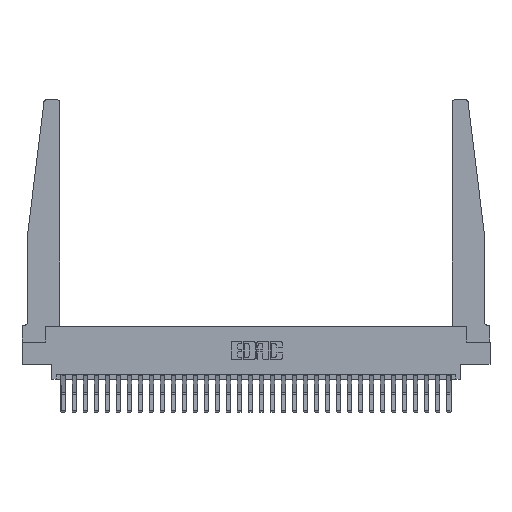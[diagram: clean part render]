
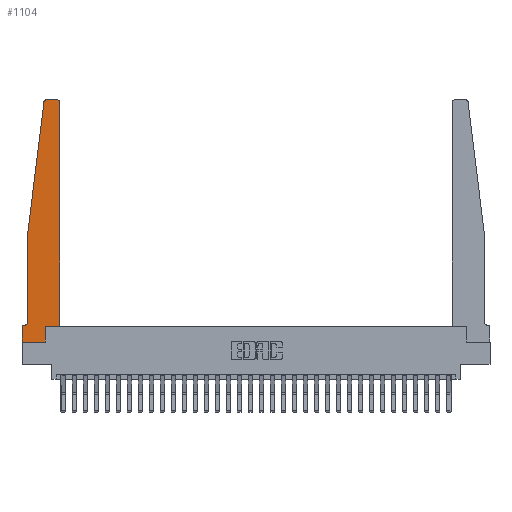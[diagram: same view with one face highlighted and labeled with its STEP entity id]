
A CAD part, top view. The second image highlights one B-rep face of the part: STEP entity #1104.
In plain terms, the highlighted planar face has unit normal (0, 0, 1).
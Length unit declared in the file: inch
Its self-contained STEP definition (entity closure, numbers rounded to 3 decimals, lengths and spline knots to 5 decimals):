
#281 = VERTEX_POINT ( 'NONE', #12625 ) ;
#428 = CARTESIAN_POINT ( 'NONE',  ( 0.425, 0.18, 0.37 ) ) ;
#993 = VECTOR ( 'NONE', #18724, 39.37008 ) ;
#1104 = ADVANCED_FACE ( 'NONE', ( #3793 ), #6349, .T. ) ;
#2392 = CARTESIAN_POINT ( 'NONE',  ( 0.425, 0.18, 0.37 ) ) ;
#2887 = VERTEX_POINT ( 'NONE', #12750 ) ;
#3393 = EDGE_CURVE ( 'NONE', #4635, #18108, #15848, .T. ) ;
#3676 = AXIS2_PLACEMENT_3D ( 'NONE', #27853, #23780, #19099 ) ;
#3747 = VERTEX_POINT ( 'NONE', #24875 ) ;
#3793 = FACE_OUTER_BOUND ( 'NONE', #11857, .T. ) ;
#3943 = DIRECTION ( 'NONE',  ( 0., 0., 1. ) ) ;
#4390 = AXIS2_PLACEMENT_3D ( 'NONE', #8921, #13291, #22461 ) ;
#4431 = CARTESIAN_POINT ( 'NONE',  ( 0.395, 2.75, 0.37 ) ) ;
#4555 = ORIENTED_EDGE ( 'NONE', *, *, #25741, .T. ) ;
#4635 = VERTEX_POINT ( 'NONE', #4431 ) ;
#4851 = ORIENTED_EDGE ( 'NONE', *, *, #26633, .T. ) ;
#4952 = LINE ( 'NONE', #2392, #10342 ) ;
#5190 = CARTESIAN_POINT ( 'NONE',  ( 0.24675, 2.72367, 0.37 ) ) ;
#5526 = EDGE_CURVE ( 'NONE', #20785, #5981, #12015, .T. ) ;
#5564 = EDGE_CURVE ( 'NONE', #19198, #20785, #4952, .T. ) ;
#5981 = VERTEX_POINT ( 'NONE', #10165 ) ;
#6349 = PLANE ( 'NONE',  #9485 ) ;
#6822 = ORIENTED_EDGE ( 'NONE', *, *, #18999, .T. ) ;
#6981 = EDGE_CURVE ( 'NONE', #5981, #4635, #8471, .T. ) ;
#7064 = ORIENTED_EDGE ( 'NONE', *, *, #13809, .T. ) ;
#7078 = CARTESIAN_POINT ( 'NONE',  ( 0., 0., 0.37 ) ) ;
#7218 = LINE ( 'NONE', #16685, #26834 ) ;
#7412 = DIRECTION ( 'NONE',  ( 0., 1., 0. ) ) ;
#7441 = VECTOR ( 'NONE', #9609, 39.37008 ) ;
#7680 = ORIENTED_EDGE ( 'NONE', *, *, #20753, .T. ) ;
#8471 = CIRCLE ( 'NONE', #21448, 0.03 ) ;
#8921 = CARTESIAN_POINT ( 'NONE',  ( 0.27653, 2.72, 0.37 ) ) ;
#9253 = CARTESIAN_POINT ( 'NONE',  ( 0.065, 0.1875, 0.37 ) ) ;
#9485 = AXIS2_PLACEMENT_3D ( 'NONE', #10552, #13115, #26671 ) ;
#9609 = DIRECTION ( 'NONE',  ( 0., 1., 0. ) ) ;
#10165 = CARTESIAN_POINT ( 'NONE',  ( 0.425, 2.72, 0.37 ) ) ;
#10342 = VECTOR ( 'NONE', #27972, 39.37008 ) ;
#10552 = CARTESIAN_POINT ( 'NONE',  ( 0., 0.1875, 0.37 ) ) ;
#10555 = VECTOR ( 'NONE', #16249, 39.37008 ) ;
#10587 = VECTOR ( 'NONE', #17979, 39.37008 ) ;
#11857 = EDGE_LOOP ( 'NONE', ( #19240, #20415, #21655, #7064, #7680, #23654, #4851, #4555, #6822, #20769, #21695, #27498 ) ) ;
#12015 = LINE ( 'NONE', #428, #7441 ) ;
#12625 = CARTESIAN_POINT ( 'NONE',  ( 0.065, 0.2375, 0.37 ) ) ;
#12696 = VERTEX_POINT ( 'NONE', #20970 ) ;
#12750 = CARTESIAN_POINT ( 'NONE',  ( 0.2605, 0., 0.37 ) ) ;
#13115 = DIRECTION ( 'NONE',  ( 0., 0., 1. ) ) ;
#13291 = DIRECTION ( 'NONE',  ( 0., 0., 1. ) ) ;
#13411 = CARTESIAN_POINT ( 'NONE',  ( 0.395, 2.72, 0.37 ) ) ;
#13669 = CARTESIAN_POINT ( 'NONE',  ( 0.27653, 2.75, 0.37 ) ) ;
#13781 = VECTOR ( 'NONE', #15879, 39.37008 ) ;
#13809 = EDGE_CURVE ( 'NONE', #14260, #281, #16159, .T. ) ;
#14064 = LINE ( 'NONE', #27769, #993 ) ;
#14260 = VERTEX_POINT ( 'NONE', #25905 ) ;
#14489 = VERTEX_POINT ( 'NONE', #16757 ) ;
#14740 = EDGE_CURVE ( 'NONE', #18108, #15865, #15899, .T. ) ;
#15848 = LINE ( 'NONE', #27013, #23288 ) ;
#15865 = VERTEX_POINT ( 'NONE', #5190 ) ;
#15879 = DIRECTION ( 'NONE',  ( -1., 0., 0. ) ) ;
#15899 = CIRCLE ( 'NONE', #4390, 0.03 ) ;
#16159 = LINE ( 'NONE', #22499, #10587 ) ;
#16249 = DIRECTION ( 'NONE',  ( 0., -1., 0. ) ) ;
#16637 = CIRCLE ( 'NONE', #3676, 0.05 ) ;
#16685 = CARTESIAN_POINT ( 'NONE',  ( 0.065, 1.25, 0.37 ) ) ;
#16757 = CARTESIAN_POINT ( 'NONE',  ( 0., 0.1875, 0.37 ) ) ;
#16879 = CARTESIAN_POINT ( 'NONE',  ( 0.2605, 0.18, 0.37 ) ) ;
#17979 = DIRECTION ( 'NONE',  ( 0., -1., 0. ) ) ;
#18108 = VERTEX_POINT ( 'NONE', #13669 ) ;
#18135 = LINE ( 'NONE', #9253, #13781 ) ;
#18724 = DIRECTION ( 'NONE',  ( 1., 0., 0. ) ) ;
#18999 = EDGE_CURVE ( 'NONE', #2887, #19198, #25777, .T. ) ;
#19099 = DIRECTION ( 'NONE',  ( -1., 0., 0. ) ) ;
#19198 = VERTEX_POINT ( 'NONE', #28633 ) ;
#19240 = ORIENTED_EDGE ( 'NONE', *, *, #3393, .T. ) ;
#20415 = ORIENTED_EDGE ( 'NONE', *, *, #14740, .T. ) ;
#20753 = EDGE_CURVE ( 'NONE', #281, #3747, #16637, .T. ) ;
#20769 = ORIENTED_EDGE ( 'NONE', *, *, #5564, .T. ) ;
#20785 = VERTEX_POINT ( 'NONE', #21368 ) ;
#20970 = CARTESIAN_POINT ( 'NONE',  ( 0., 0., 0.37 ) ) ;
#21368 = CARTESIAN_POINT ( 'NONE',  ( 0.425, 0.18, 0.37 ) ) ;
#21448 = AXIS2_PLACEMENT_3D ( 'NONE', #13411, #3943, #22140 ) ;
#21483 = EDGE_CURVE ( 'NONE', #3747, #14489, #18135, .T. ) ;
#21655 = ORIENTED_EDGE ( 'NONE', *, *, #23556, .T. ) ;
#21695 = ORIENTED_EDGE ( 'NONE', *, *, #5526, .T. ) ;
#22140 = DIRECTION ( 'NONE',  ( 1., 0., 0. ) ) ;
#22461 = DIRECTION ( 'NONE',  ( 1., 0., 0. ) ) ;
#22499 = CARTESIAN_POINT ( 'NONE',  ( 0.065, 1.25, 0.37 ) ) ;
#23288 = VECTOR ( 'NONE', #29114, 39.37008 ) ;
#23556 = EDGE_CURVE ( 'NONE', #15865, #14260, #7218, .T. ) ;
#23654 = ORIENTED_EDGE ( 'NONE', *, *, #21483, .T. ) ;
#23780 = DIRECTION ( 'NONE',  ( 0., 0., -1. ) ) ;
#24875 = CARTESIAN_POINT ( 'NONE',  ( 0.015, 0.1875, 0.37 ) ) ;
#25291 = DIRECTION ( 'NONE',  ( -0.122, -0.992, 0. ) ) ;
#25294 = VECTOR ( 'NONE', #7412, 39.37008 ) ;
#25741 = EDGE_CURVE ( 'NONE', #12696, #2887, #14064, .T. ) ;
#25777 = LINE ( 'NONE', #16879, #25294 ) ;
#25905 = CARTESIAN_POINT ( 'NONE',  ( 0.065, 1.25, 0.37 ) ) ;
#26633 = EDGE_CURVE ( 'NONE', #14489, #12696, #27267, .T. ) ;
#26671 = DIRECTION ( 'NONE',  ( 1., 0., 0. ) ) ;
#26834 = VECTOR ( 'NONE', #25291, 39.37008 ) ;
#27013 = CARTESIAN_POINT ( 'NONE',  ( 0.25, 2.75, 0.37 ) ) ;
#27267 = LINE ( 'NONE', #7078, #10555 ) ;
#27498 = ORIENTED_EDGE ( 'NONE', *, *, #6981, .T. ) ;
#27769 = CARTESIAN_POINT ( 'NONE',  ( 0., 0., 0.37 ) ) ;
#27853 = CARTESIAN_POINT ( 'NONE',  ( 0.015, 0.2375, 0.37 ) ) ;
#27972 = DIRECTION ( 'NONE',  ( 1., 0., 0. ) ) ;
#28633 = CARTESIAN_POINT ( 'NONE',  ( 0.2605, 0.18, 0.37 ) ) ;
#29114 = DIRECTION ( 'NONE',  ( -1., 0., 0. ) ) ;
